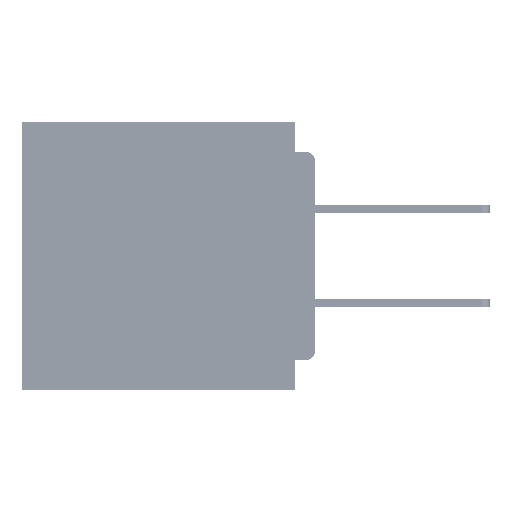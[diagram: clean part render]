
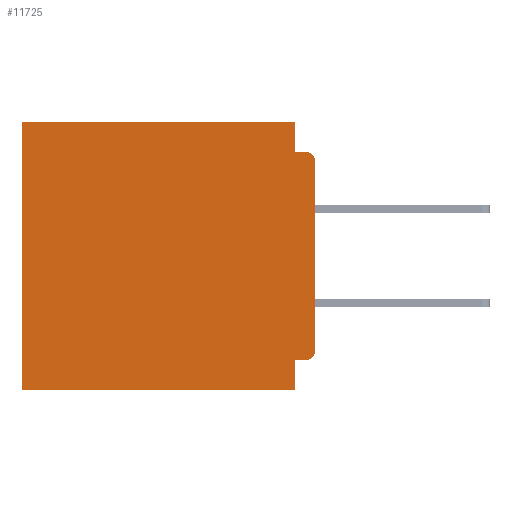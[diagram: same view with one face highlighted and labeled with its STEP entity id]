
A CAD part, left-side view. The second image highlights one B-rep face of the part: STEP entity #11725.
In plain terms, the highlighted planar face has unit normal (-1, 0, 0).
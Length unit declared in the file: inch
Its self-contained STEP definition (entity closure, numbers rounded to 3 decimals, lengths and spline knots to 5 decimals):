
#413 = LINE ( 'NONE', #5363, #27126 ) ;
#2671 = ORIENTED_EDGE ( 'NONE', *, *, #62720, .F. ) ;
#2952 = VECTOR ( 'NONE', #34303, 39.37008 ) ;
#3411 = DIRECTION ( 'NONE',  ( 0., 1., 0. ) ) ;
#3766 = EDGE_CURVE ( 'NONE', #61323, #47820, #42590, .T. ) ;
#4707 = LINE ( 'NONE', #39847, #17197 ) ;
#4885 = CARTESIAN_POINT ( 'NONE',  ( 0.3, 0.015, -0.355 ) ) ;
#5363 = CARTESIAN_POINT ( 'NONE',  ( 0.3, 0., -0.4 ) ) ;
#5643 = CARTESIAN_POINT ( 'NONE',  ( 0.3, 0.031, -0.355 ) ) ;
#7105 = DIRECTION ( 'NONE',  ( 0., 0., -1. ) ) ;
#7415 = CARTESIAN_POINT ( 'NONE',  ( 0.3, 0., -0.045 ) ) ;
#8269 = VERTEX_POINT ( 'NONE', #11658 ) ;
#9121 = CIRCLE ( 'NONE', #18116, 0.015 ) ;
#9809 = EDGE_CURVE ( 'NONE', #58421, #58167, #9121, .T. ) ;
#11658 = CARTESIAN_POINT ( 'NONE',  ( 0.3, 0.031, -0.045 ) ) ;
#11725 = ADVANCED_FACE ( 'NONE', ( #58660 ), #33587, .F. ) ;
#12354 = CARTESIAN_POINT ( 'NONE',  ( 0.3, 0., -0.355 ) ) ;
#16006 = AXIS2_PLACEMENT_3D ( 'NONE', #22881, #38876, #7105 ) ;
#16124 = CARTESIAN_POINT ( 'NONE',  ( 0.3, 0.031, 0. ) ) ;
#16265 = EDGE_CURVE ( 'NONE', #8269, #58167, #23752, .T. ) ;
#17142 = LINE ( 'NONE', #28994, #2952 ) ;
#17197 = VECTOR ( 'NONE', #34549, 39.37008 ) ;
#17666 = DIRECTION ( 'NONE',  ( 0., 1., 0. ) ) ;
#18116 = AXIS2_PLACEMENT_3D ( 'NONE', #50813, #19073, #56171 ) ;
#18332 = ORIENTED_EDGE ( 'NONE', *, *, #3766, .F. ) ;
#19073 = DIRECTION ( 'NONE',  ( -1., 0., 0. ) ) ;
#20765 = EDGE_CURVE ( 'NONE', #27405, #8269, #56900, .T. ) ;
#21295 = CARTESIAN_POINT ( 'NONE',  ( 0.3, 0., -0.4 ) ) ;
#21309 = VECTOR ( 'NONE', #57037, 39.37008 ) ;
#22881 = CARTESIAN_POINT ( 'NONE',  ( 0.3, 0., -0.4 ) ) ;
#23752 = LINE ( 'NONE', #7415, #37873 ) ;
#24087 = CARTESIAN_POINT ( 'NONE',  ( 0.3, 0.015, -0.34 ) ) ;
#24971 = AXIS2_PLACEMENT_3D ( 'NONE', #24087, #61211, #29462 ) ;
#25014 = CARTESIAN_POINT ( 'NONE',  ( 0.3, 0., 0. ) ) ;
#26261 = EDGE_CURVE ( 'NONE', #44911, #47820, #4707, .T. ) ;
#26399 = EDGE_CURVE ( 'NONE', #27405, #44911, #51154, .T. ) ;
#27126 = VECTOR ( 'NONE', #47788, 39.37008 ) ;
#27281 = VERTEX_POINT ( 'NONE', #5643 ) ;
#27405 = VERTEX_POINT ( 'NONE', #27929 ) ;
#27929 = CARTESIAN_POINT ( 'NONE',  ( 0.3, 0.031, 0. ) ) ;
#28668 = VERTEX_POINT ( 'NONE', #37228 ) ;
#28711 = VECTOR ( 'NONE', #47821, 39.37008 ) ;
#28994 = CARTESIAN_POINT ( 'NONE',  ( 0.3, 0.031, -0.4 ) ) ;
#29462 = DIRECTION ( 'NONE',  ( 0., 0., -1. ) ) ;
#29963 = ORIENTED_EDGE ( 'NONE', *, *, #42638, .T. ) ;
#31712 = ORIENTED_EDGE ( 'NONE', *, *, #20765, .F. ) ;
#33587 = PLANE ( 'NONE',  #16006 ) ;
#34303 = DIRECTION ( 'NONE',  ( 0., 0., -1. ) ) ;
#34549 = DIRECTION ( 'NONE',  ( 0., 0., -1. ) ) ;
#35258 = ORIENTED_EDGE ( 'NONE', *, *, #26261, .T. ) ;
#35737 = CARTESIAN_POINT ( 'NONE',  ( 0.3, 0., -0.06 ) ) ;
#36382 = ORIENTED_EDGE ( 'NONE', *, *, #37991, .F. ) ;
#37228 = CARTESIAN_POINT ( 'NONE',  ( 0.3, 0., -0.34 ) ) ;
#37873 = VECTOR ( 'NONE', #60544, 39.37008 ) ;
#37991 = EDGE_CURVE ( 'NONE', #58421, #28668, #413, .T. ) ;
#38876 = DIRECTION ( 'NONE',  ( 1., 0., 0. ) ) ;
#39224 = ORIENTED_EDGE ( 'NONE', *, *, #45802, .F. ) ;
#39847 = CARTESIAN_POINT ( 'NONE',  ( 0.3, 0.437, -0.4 ) ) ;
#40308 = VERTEX_POINT ( 'NONE', #4885 ) ;
#41130 = LINE ( 'NONE', #12354, #67708 ) ;
#41427 = CARTESIAN_POINT ( 'NONE',  ( 0.3, 0.437, -0.4 ) ) ;
#42590 = LINE ( 'NONE', #21295, #55021 ) ;
#42638 = EDGE_CURVE ( 'NONE', #40308, #28668, #44665, .T. ) ;
#44665 = CIRCLE ( 'NONE', #24971, 0.015 ) ;
#44878 = ORIENTED_EDGE ( 'NONE', *, *, #26399, .T. ) ;
#44911 = VERTEX_POINT ( 'NONE', #63010 ) ;
#45802 = EDGE_CURVE ( 'NONE', #40308, #27281, #41130, .T. ) ;
#47788 = DIRECTION ( 'NONE',  ( 0., 0., -1. ) ) ;
#47820 = VERTEX_POINT ( 'NONE', #41427 ) ;
#47821 = DIRECTION ( 'NONE',  ( 0., 0., -1. ) ) ;
#49898 = CARTESIAN_POINT ( 'NONE',  ( 0.3, 0.015, -0.045 ) ) ;
#50813 = CARTESIAN_POINT ( 'NONE',  ( 0.3, 0.015, -0.06 ) ) ;
#51154 = LINE ( 'NONE', #25014, #21309 ) ;
#55021 = VECTOR ( 'NONE', #3411, 39.37008 ) ;
#56171 = DIRECTION ( 'NONE',  ( 0., 0., -1. ) ) ;
#56900 = LINE ( 'NONE', #16124, #28711 ) ;
#57037 = DIRECTION ( 'NONE',  ( 0., 1., 0. ) ) ;
#58167 = VERTEX_POINT ( 'NONE', #49898 ) ;
#58421 = VERTEX_POINT ( 'NONE', #35737 ) ;
#58660 = FACE_OUTER_BOUND ( 'NONE', #59245, .T. ) ;
#59245 = EDGE_LOOP ( 'NONE', ( #36382, #65312, #65574, #31712, #44878, #35258, #18332, #2671, #39224, #29963 ) ) ;
#60544 = DIRECTION ( 'NONE',  ( 0., -1., 0. ) ) ;
#61211 = DIRECTION ( 'NONE',  ( -1., 0., 0. ) ) ;
#61323 = VERTEX_POINT ( 'NONE', #64624 ) ;
#62720 = EDGE_CURVE ( 'NONE', #27281, #61323, #17142, .T. ) ;
#63010 = CARTESIAN_POINT ( 'NONE',  ( 0.3, 0.437, 0. ) ) ;
#64624 = CARTESIAN_POINT ( 'NONE',  ( 0.3, 0.031, -0.4 ) ) ;
#65312 = ORIENTED_EDGE ( 'NONE', *, *, #9809, .T. ) ;
#65574 = ORIENTED_EDGE ( 'NONE', *, *, #16265, .F. ) ;
#67708 = VECTOR ( 'NONE', #17666, 39.37008 ) ;
